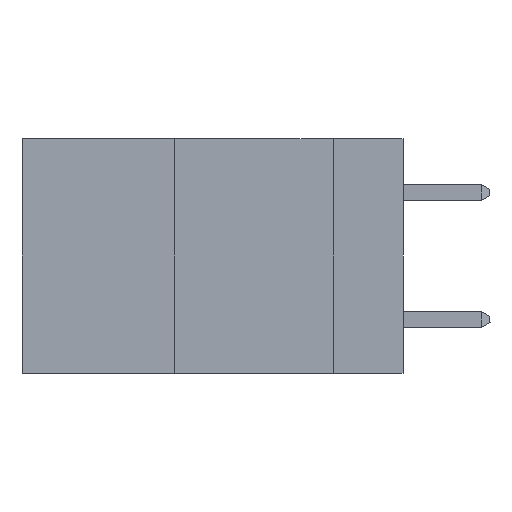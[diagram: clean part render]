
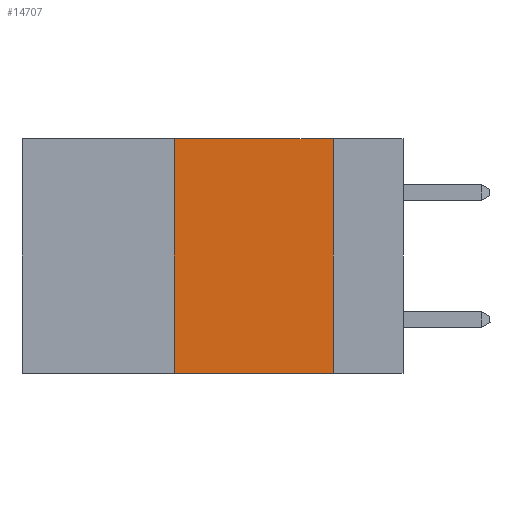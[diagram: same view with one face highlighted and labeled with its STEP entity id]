
A CAD part, left-side view. The second image highlights one B-rep face of the part: STEP entity #14707.
In plain terms, the highlighted planar face has unit normal (-1, 0, 0).
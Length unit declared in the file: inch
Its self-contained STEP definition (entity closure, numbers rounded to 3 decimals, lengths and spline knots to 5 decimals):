
#125 = FACE_OUTER_BOUND ( 'NONE', #10996, .T. ) ;
#2226 = EDGE_CURVE ( 'NONE', #24907, #2702, #22624, .T. ) ;
#2310 = EDGE_CURVE ( 'NONE', #10003, #24907, #3398, .T. ) ;
#2702 = VERTEX_POINT ( 'NONE', #31636 ) ;
#3398 = LINE ( 'NONE', #10667, #15970 ) ;
#4806 = CARTESIAN_POINT ( 'NONE',  ( 0., 0.11, 0. ) ) ;
#5132 = ORIENTED_EDGE ( 'NONE', *, *, #2310, .F. ) ;
#5358 = EDGE_CURVE ( 'NONE', #8912, #2702, #31937, .T. ) ;
#5598 = DIRECTION ( 'NONE',  ( 0., 0., 1. ) ) ;
#7678 = DIRECTION ( 'NONE',  ( 0., 0., -1. ) ) ;
#7822 = CARTESIAN_POINT ( 'NONE',  ( 0., 0.36, 0. ) ) ;
#8912 = VERTEX_POINT ( 'NONE', #18442 ) ;
#9575 = VECTOR ( 'NONE', #31346, 39.37008 ) ;
#10003 = VERTEX_POINT ( 'NONE', #18728 ) ;
#10667 = CARTESIAN_POINT ( 'NONE',  ( 0., 0.6, 0. ) ) ;
#10996 = EDGE_LOOP ( 'NONE', ( #26822, #5132, #32277, #23317 ) ) ;
#12751 = DIRECTION ( 'NONE',  ( 1., 0., 0. ) ) ;
#14707 = ADVANCED_FACE ( 'NONE', ( #125 ), #20980, .F. ) ;
#15661 = DIRECTION ( 'NONE',  ( 0., -1., 0. ) ) ;
#15970 = VECTOR ( 'NONE', #15661, 39.37008 ) ;
#18055 = CARTESIAN_POINT ( 'NONE',  ( 0., 0.11, 0. ) ) ;
#18298 = EDGE_CURVE ( 'NONE', #8912, #10003, #30925, .T. ) ;
#18340 = VECTOR ( 'NONE', #7678, 39.37008 ) ;
#18442 = CARTESIAN_POINT ( 'NONE',  ( 0., 0.36, -0.37 ) ) ;
#18728 = CARTESIAN_POINT ( 'NONE',  ( 0., 0.36, 0. ) ) ;
#19607 = AXIS2_PLACEMENT_3D ( 'NONE', #30997, #12751, #25064 ) ;
#20980 = PLANE ( 'NONE',  #19607 ) ;
#21952 = VECTOR ( 'NONE', #5598, 39.37008 ) ;
#22624 = LINE ( 'NONE', #4806, #18340 ) ;
#23317 = ORIENTED_EDGE ( 'NONE', *, *, #5358, .T. ) ;
#24907 = VERTEX_POINT ( 'NONE', #18055 ) ;
#25064 = DIRECTION ( 'NONE',  ( 0., 0., -1. ) ) ;
#26300 = CARTESIAN_POINT ( 'NONE',  ( 0., 0.6, -0.37 ) ) ;
#26822 = ORIENTED_EDGE ( 'NONE', *, *, #2226, .F. ) ;
#30925 = LINE ( 'NONE', #7822, #21952 ) ;
#30997 = CARTESIAN_POINT ( 'NONE',  ( 0., 0.6, 0. ) ) ;
#31346 = DIRECTION ( 'NONE',  ( 0., -1., 0. ) ) ;
#31636 = CARTESIAN_POINT ( 'NONE',  ( 0., 0.11, -0.37 ) ) ;
#31937 = LINE ( 'NONE', #26300, #9575 ) ;
#32277 = ORIENTED_EDGE ( 'NONE', *, *, #18298, .F. ) ;
